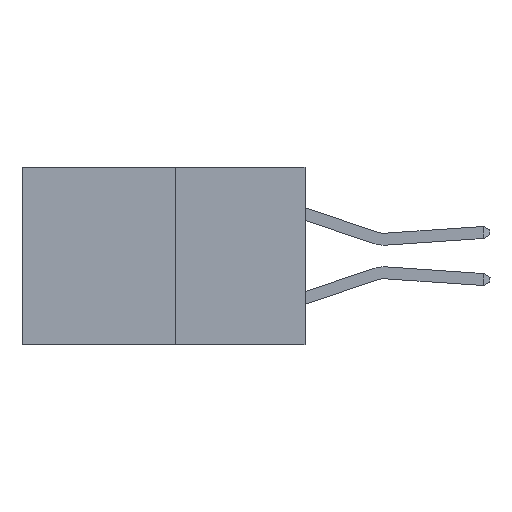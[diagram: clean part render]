
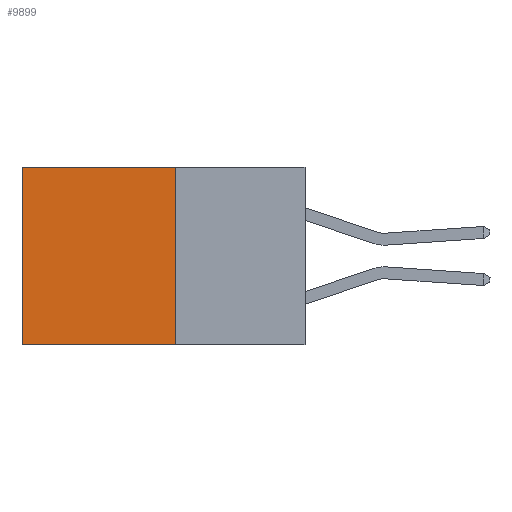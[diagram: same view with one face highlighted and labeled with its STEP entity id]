
A CAD part, left-side view. The second image highlights one B-rep face of the part: STEP entity #9899.
In plain terms, the highlighted planar face has unit normal (-1, 0, 0).
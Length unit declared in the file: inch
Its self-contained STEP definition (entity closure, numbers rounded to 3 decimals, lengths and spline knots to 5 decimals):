
#616 = ORIENTED_EDGE ( 'NONE', *, *, #15413, .F. ) ;
#737 = EDGE_LOOP ( 'NONE', ( #12171, #15895, #616, #7090 ) ) ;
#994 = VECTOR ( 'NONE', #1859, 39.37008 ) ;
#1427 = AXIS2_PLACEMENT_3D ( 'NONE', #3848, #1769, #1728 ) ;
#1455 = LINE ( 'NONE', #13202, #994 ) ;
#1728 = DIRECTION ( 'NONE',  ( 0., 0., -1. ) ) ;
#1769 = DIRECTION ( 'NONE',  ( 1., 0., 0. ) ) ;
#1859 = DIRECTION ( 'NONE',  ( 0., 1., 0. ) ) ;
#1880 = VECTOR ( 'NONE', #17249, 39.37008 ) ;
#2128 = PLANE ( 'NONE',  #1427 ) ;
#2175 = LINE ( 'NONE', #3379, #5981 ) ;
#3379 = CARTESIAN_POINT ( 'NONE',  ( 0.277, 0.27, -0.37 ) ) ;
#3848 = CARTESIAN_POINT ( 'NONE',  ( 0.277, 0.27, -0.37 ) ) ;
#4172 = CARTESIAN_POINT ( 'NONE',  ( 0.277, 0.59, -0.37 ) ) ;
#5079 = VERTEX_POINT ( 'NONE', #4172 ) ;
#5208 = FACE_OUTER_BOUND ( 'NONE', #737, .T. ) ;
#5981 = VECTOR ( 'NONE', #16056, 39.37008 ) ;
#7090 = ORIENTED_EDGE ( 'NONE', *, *, #8271, .T. ) ;
#8271 = EDGE_CURVE ( 'NONE', #10707, #11993, #15866, .T. ) ;
#9348 = EDGE_CURVE ( 'NONE', #11993, #5079, #13639, .T. ) ;
#9899 = ADVANCED_FACE ( 'NONE', ( #5208 ), #2128, .F. ) ;
#10493 = VERTEX_POINT ( 'NONE', #16588 ) ;
#10616 = EDGE_CURVE ( 'NONE', #10493, #5079, #1455, .T. ) ;
#10707 = VERTEX_POINT ( 'NONE', #15583 ) ;
#11993 = VERTEX_POINT ( 'NONE', #17090 ) ;
#12144 = VECTOR ( 'NONE', #12190, 39.37008 ) ;
#12171 = ORIENTED_EDGE ( 'NONE', *, *, #9348, .T. ) ;
#12190 = DIRECTION ( 'NONE',  ( 0., 1., 0. ) ) ;
#12856 = CARTESIAN_POINT ( 'NONE',  ( 0.277, 0.27, 0. ) ) ;
#13202 = CARTESIAN_POINT ( 'NONE',  ( 0.277, 0.27, -0.37 ) ) ;
#13639 = LINE ( 'NONE', #17342, #1880 ) ;
#15413 = EDGE_CURVE ( 'NONE', #10707, #10493, #2175, .T. ) ;
#15583 = CARTESIAN_POINT ( 'NONE',  ( 0.277, 0.27, 0. ) ) ;
#15866 = LINE ( 'NONE', #12856, #12144 ) ;
#15895 = ORIENTED_EDGE ( 'NONE', *, *, #10616, .F. ) ;
#16056 = DIRECTION ( 'NONE',  ( 0., 0., -1. ) ) ;
#16588 = CARTESIAN_POINT ( 'NONE',  ( 0.277, 0.27, -0.37 ) ) ;
#17090 = CARTESIAN_POINT ( 'NONE',  ( 0.277, 0.59, 0. ) ) ;
#17249 = DIRECTION ( 'NONE',  ( 0., 0., -1. ) ) ;
#17342 = CARTESIAN_POINT ( 'NONE',  ( 0.277, 0.59, -0.37 ) ) ;
